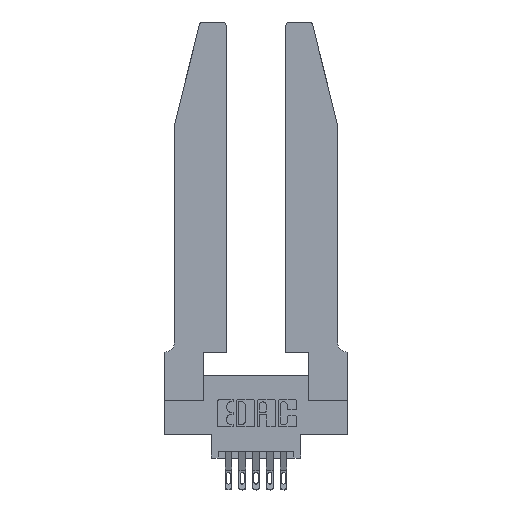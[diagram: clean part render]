
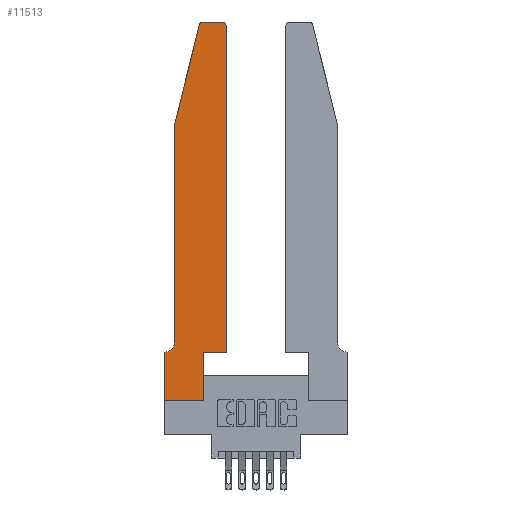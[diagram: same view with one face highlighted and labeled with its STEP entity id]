
A CAD part, top view. The second image highlights one B-rep face of the part: STEP entity #11513.
In plain terms, the highlighted planar face has unit normal (0, 0, 1).
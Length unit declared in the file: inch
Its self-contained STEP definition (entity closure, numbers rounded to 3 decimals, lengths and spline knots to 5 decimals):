
#198 = CARTESIAN_POINT ( 'NONE',  ( 0.0755, 0.35, 0.37 ) ) ;
#263 = VERTEX_POINT ( 'NONE', #7269 ) ;
#324 = DIRECTION ( 'NONE',  ( 0., 0., 1. ) ) ;
#528 = EDGE_CURVE ( 'NONE', #11684, #8623, #13932, .T. ) ;
#547 = LINE ( 'NONE', #10157, #3347 ) ;
#944 = VECTOR ( 'NONE', #1430, 39.37008 ) ;
#967 = DIRECTION ( 'NONE',  ( 0., 0., 1. ) ) ;
#1090 = ORIENTED_EDGE ( 'NONE', *, *, #10503, .T. ) ;
#1110 = AXIS2_PLACEMENT_3D ( 'NONE', #2072, #11780, #8468 ) ;
#1193 = ORIENTED_EDGE ( 'NONE', *, *, #2691, .T. ) ;
#1430 = DIRECTION ( 'NONE',  ( -1., 0., 0. ) ) ;
#1460 = CARTESIAN_POINT ( 'NONE',  ( 0., 0., 0.37 ) ) ;
#1600 = ORIENTED_EDGE ( 'NONE', *, *, #528, .T. ) ;
#1613 = LINE ( 'NONE', #11680, #10401 ) ;
#1751 = VECTOR ( 'NONE', #12834, 39.37008 ) ;
#1856 = EDGE_LOOP ( 'NONE', ( #5312, #5518, #10286, #1090, #13282, #10151, #2593, #11209, #7176, #1193, #4387, #1600 ) ) ;
#2072 = CARTESIAN_POINT ( 'NONE',  ( 0.4205, 2.72, 0.37 ) ) ;
#2138 = DIRECTION ( 'NONE',  ( 0., 0., -1. ) ) ;
#2325 = VERTEX_POINT ( 'NONE', #13884 ) ;
#2375 = CARTESIAN_POINT ( 'NONE',  ( 0.284, 2.75, 0.37 ) ) ;
#2392 = VERTEX_POINT ( 'NONE', #13976 ) ;
#2593 = ORIENTED_EDGE ( 'NONE', *, *, #10262, .T. ) ;
#2632 = VERTEX_POINT ( 'NONE', #4856 ) ;
#2691 = EDGE_CURVE ( 'NONE', #2714, #5370, #12140, .T. ) ;
#2711 = LINE ( 'NONE', #8323, #13726 ) ;
#2714 = VERTEX_POINT ( 'NONE', #12423 ) ;
#2750 = CARTESIAN_POINT ( 'NONE',  ( 0.0755, 2., 0.37 ) ) ;
#2907 = AXIS2_PLACEMENT_3D ( 'NONE', #7731, #967, #8816 ) ;
#3347 = VECTOR ( 'NONE', #10115, 39.37008 ) ;
#3480 = CARTESIAN_POINT ( 'NONE',  ( 0.4505, 0.35, 0.37 ) ) ;
#3771 = VERTEX_POINT ( 'NONE', #2750 ) ;
#3840 = CARTESIAN_POINT ( 'NONE',  ( 0., 0., 0.37 ) ) ;
#4178 = DIRECTION ( 'NONE',  ( 0., 1., 0. ) ) ;
#4387 = ORIENTED_EDGE ( 'NONE', *, *, #5940, .T. ) ;
#4626 = LINE ( 'NONE', #3840, #10034 ) ;
#4856 = CARTESIAN_POINT ( 'NONE',  ( 0.0055, 0.35, 0.37 ) ) ;
#5073 = LINE ( 'NONE', #6817, #7625 ) ;
#5266 = EDGE_CURVE ( 'NONE', #2392, #2632, #11758, .T. ) ;
#5312 = ORIENTED_EDGE ( 'NONE', *, *, #13516, .T. ) ;
#5370 = VERTEX_POINT ( 'NONE', #3480 ) ;
#5470 = CARTESIAN_POINT ( 'NONE',  ( 0.0755, 2., 0.37 ) ) ;
#5518 = ORIENTED_EDGE ( 'NONE', *, *, #8257, .T. ) ;
#5603 = VERTEX_POINT ( 'NONE', #6081 ) ;
#5720 = DIRECTION ( 'NONE',  ( 0., 1., 0. ) ) ;
#5940 = EDGE_CURVE ( 'NONE', #5370, #11684, #5073, .T. ) ;
#6038 = VECTOR ( 'NONE', #13375, 39.37008 ) ;
#6068 = PLANE ( 'NONE',  #13811 ) ;
#6069 = DIRECTION ( 'NONE',  ( 1., 0., 0. ) ) ;
#6081 = CARTESIAN_POINT ( 'NONE',  ( 0.2865, 0., 0.37 ) ) ;
#6344 = CARTESIAN_POINT ( 'NONE',  ( 0.4505, 2.72, 0.37 ) ) ;
#6662 = CARTESIAN_POINT ( 'NONE',  ( 0.25487, 2.72718, 0.37 ) ) ;
#6817 = CARTESIAN_POINT ( 'NONE',  ( 0.4505, 0.35, 0.37 ) ) ;
#7176 = ORIENTED_EDGE ( 'NONE', *, *, #8713, .T. ) ;
#7269 = CARTESIAN_POINT ( 'NONE',  ( 0., 0., 0.37 ) ) ;
#7344 = VECTOR ( 'NONE', #6069, 39.37008 ) ;
#7625 = VECTOR ( 'NONE', #5720, 39.37008 ) ;
#7731 = CARTESIAN_POINT ( 'NONE',  ( 0.284, 2.72, 0.37 ) ) ;
#8230 = DIRECTION ( 'NONE',  ( 1., 0., 0. ) ) ;
#8257 = EDGE_CURVE ( 'NONE', #12947, #10569, #10419, .T. ) ;
#8278 = DIRECTION ( 'NONE',  ( -0.239, -0.971, 0. ) ) ;
#8323 = CARTESIAN_POINT ( 'NONE',  ( 0.0755, 2., 0.37 ) ) ;
#8468 = DIRECTION ( 'NONE',  ( 1., 0., 0. ) ) ;
#8623 = VERTEX_POINT ( 'NONE', #13582 ) ;
#8713 = EDGE_CURVE ( 'NONE', #5603, #2714, #1613, .T. ) ;
#8770 = CARTESIAN_POINT ( 'NONE',  ( 0.0055, 0.42, 0.37 ) ) ;
#8816 = DIRECTION ( 'NONE',  ( 1., 0., 0. ) ) ;
#8900 = LINE ( 'NONE', #1460, #6038 ) ;
#9164 = EDGE_CURVE ( 'NONE', #10569, #3771, #2711, .T. ) ;
#9184 = FACE_OUTER_BOUND ( 'NONE', #1856, .T. ) ;
#9260 = DIRECTION ( 'NONE',  ( 0., -1., 0. ) ) ;
#9606 = EDGE_CURVE ( 'NONE', #263, #5603, #8900, .T. ) ;
#9834 = DIRECTION ( 'NONE',  ( -1., 0., 0. ) ) ;
#9841 = LINE ( 'NONE', #198, #944 ) ;
#10034 = VECTOR ( 'NONE', #9260, 39.37008 ) ;
#10115 = DIRECTION ( 'NONE',  ( -1., 0., 0. ) ) ;
#10151 = ORIENTED_EDGE ( 'NONE', *, *, #11469, .T. ) ;
#10157 = CARTESIAN_POINT ( 'NONE',  ( 0.2605, 2.75, 0.37 ) ) ;
#10262 = EDGE_CURVE ( 'NONE', #2325, #263, #4626, .T. ) ;
#10286 = ORIENTED_EDGE ( 'NONE', *, *, #9164, .T. ) ;
#10401 = VECTOR ( 'NONE', #4178, 39.37008 ) ;
#10419 = CIRCLE ( 'NONE', #2907, 0.03 ) ;
#10503 = EDGE_CURVE ( 'NONE', #3771, #2392, #12598, .T. ) ;
#10569 = VERTEX_POINT ( 'NONE', #6662 ) ;
#10858 = AXIS2_PLACEMENT_3D ( 'NONE', #8770, #2138, #9834 ) ;
#11209 = ORIENTED_EDGE ( 'NONE', *, *, #9606, .T. ) ;
#11469 = EDGE_CURVE ( 'NONE', #2632, #2325, #9841, .T. ) ;
#11513 = ADVANCED_FACE ( 'NONE', ( #9184 ), #6068, .T. ) ;
#11680 = CARTESIAN_POINT ( 'NONE',  ( 0.2865, 0.35, 0.37 ) ) ;
#11684 = VERTEX_POINT ( 'NONE', #6344 ) ;
#11758 = CIRCLE ( 'NONE', #10858, 0.07 ) ;
#11780 = DIRECTION ( 'NONE',  ( 0., 0., 1. ) ) ;
#12140 = LINE ( 'NONE', #13394, #7344 ) ;
#12423 = CARTESIAN_POINT ( 'NONE',  ( 0.2865, 0.35, 0.37 ) ) ;
#12598 = LINE ( 'NONE', #5470, #1751 ) ;
#12834 = DIRECTION ( 'NONE',  ( 0., -1., 0. ) ) ;
#12947 = VERTEX_POINT ( 'NONE', #2375 ) ;
#13282 = ORIENTED_EDGE ( 'NONE', *, *, #5266, .T. ) ;
#13375 = DIRECTION ( 'NONE',  ( 1., 0., 0. ) ) ;
#13392 = CARTESIAN_POINT ( 'NONE',  ( 0., 0.35, 0.37 ) ) ;
#13394 = CARTESIAN_POINT ( 'NONE',  ( 0.4505, 0.35, 0.37 ) ) ;
#13516 = EDGE_CURVE ( 'NONE', #8623, #12947, #547, .T. ) ;
#13582 = CARTESIAN_POINT ( 'NONE',  ( 0.4205, 2.75, 0.37 ) ) ;
#13726 = VECTOR ( 'NONE', #8278, 39.37008 ) ;
#13811 = AXIS2_PLACEMENT_3D ( 'NONE', #13392, #324, #8230 ) ;
#13884 = CARTESIAN_POINT ( 'NONE',  ( 0., 0.35, 0.37 ) ) ;
#13932 = CIRCLE ( 'NONE', #1110, 0.03 ) ;
#13976 = CARTESIAN_POINT ( 'NONE',  ( 0.0755, 0.42, 0.37 ) ) ;
